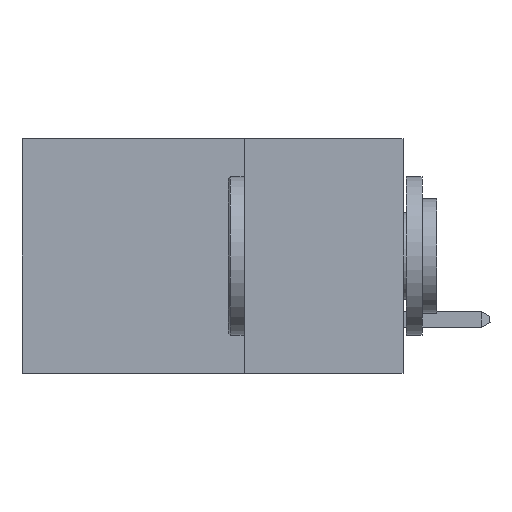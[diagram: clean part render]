
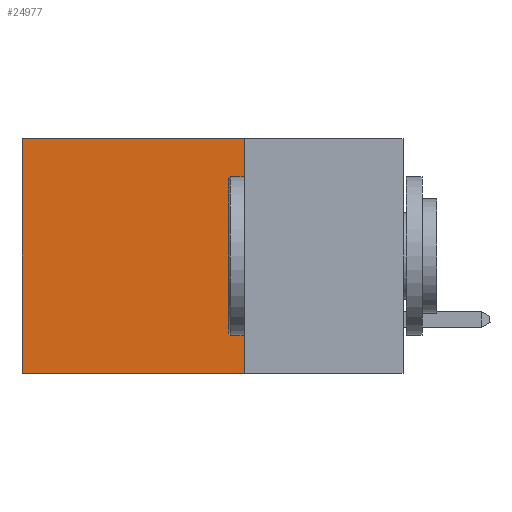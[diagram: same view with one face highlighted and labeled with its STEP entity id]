
A CAD part, left-side view. The second image highlights one B-rep face of the part: STEP entity #24977.
In plain terms, the highlighted planar face has unit normal (-1, 0, 0).
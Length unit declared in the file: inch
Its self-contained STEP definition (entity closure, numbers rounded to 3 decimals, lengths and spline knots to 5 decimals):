
#1694 = CARTESIAN_POINT ( 'NONE',  ( 0.2875, 0.6, 0. ) ) ;
#1926 = EDGE_CURVE ( 'NONE', #26159, #25544, #29488, .T. ) ;
#2100 = AXIS2_PLACEMENT_3D ( 'NONE', #13046, #10799, #15730 ) ;
#2441 = FACE_OUTER_BOUND ( 'NONE', #2463, .T. ) ;
#2463 = EDGE_LOOP ( 'NONE', ( #6213, #17209, #7531, #12561 ) ) ;
#2525 = PLANE ( 'NONE',  #2100 ) ;
#2778 = CARTESIAN_POINT ( 'NONE',  ( 0.2875, 0.6, -0.37 ) ) ;
#3217 = EDGE_CURVE ( 'NONE', #23354, #26159, #5115, .T. ) ;
#4455 = VECTOR ( 'NONE', #12534, 39.37008 ) ;
#4984 = EDGE_CURVE ( 'NONE', #25813, #25544, #27620, .T. ) ;
#5115 = LINE ( 'NONE', #22896, #5523 ) ;
#5523 = VECTOR ( 'NONE', #28778, 39.37008 ) ;
#6213 = ORIENTED_EDGE ( 'NONE', *, *, #4984, .T. ) ;
#7208 = EDGE_CURVE ( 'NONE', #23354, #25813, #27907, .T. ) ;
#7509 = VECTOR ( 'NONE', #21911, 39.37008 ) ;
#7531 = ORIENTED_EDGE ( 'NONE', *, *, #3217, .F. ) ;
#9911 = CARTESIAN_POINT ( 'NONE',  ( 0.2875, 0.6, 0. ) ) ;
#10799 = DIRECTION ( 'NONE',  ( 1., 0., 0. ) ) ;
#11289 = CARTESIAN_POINT ( 'NONE',  ( 0.2875, 0.25, -0.37 ) ) ;
#12534 = DIRECTION ( 'NONE',  ( 0., 1., 0. ) ) ;
#12561 = ORIENTED_EDGE ( 'NONE', *, *, #7208, .T. ) ;
#13046 = CARTESIAN_POINT ( 'NONE',  ( 0.2875, 0.25, 0. ) ) ;
#15730 = DIRECTION ( 'NONE',  ( 0., 0., -1. ) ) ;
#17209 = ORIENTED_EDGE ( 'NONE', *, *, #1926, .F. ) ;
#17318 = CARTESIAN_POINT ( 'NONE',  ( 0.2875, 0.25, 0. ) ) ;
#21911 = DIRECTION ( 'NONE',  ( 0., 0., -1. ) ) ;
#22896 = CARTESIAN_POINT ( 'NONE',  ( 0.2875, 0.25, 0. ) ) ;
#23354 = VERTEX_POINT ( 'NONE', #32966 ) ;
#24977 = ADVANCED_FACE ( 'NONE', ( #2441 ), #2525, .F. ) ;
#25544 = VERTEX_POINT ( 'NONE', #2778 ) ;
#25813 = VERTEX_POINT ( 'NONE', #1694 ) ;
#26159 = VERTEX_POINT ( 'NONE', #26625 ) ;
#26625 = CARTESIAN_POINT ( 'NONE',  ( 0.2875, 0.25, -0.37 ) ) ;
#27620 = LINE ( 'NONE', #9911, #7509 ) ;
#27907 = LINE ( 'NONE', #17318, #4455 ) ;
#28778 = DIRECTION ( 'NONE',  ( 0., 0., -1. ) ) ;
#29488 = LINE ( 'NONE', #11289, #34143 ) ;
#30047 = DIRECTION ( 'NONE',  ( 0., 1., 0. ) ) ;
#32966 = CARTESIAN_POINT ( 'NONE',  ( 0.2875, 0.25, 0. ) ) ;
#34143 = VECTOR ( 'NONE', #30047, 39.37008 ) ;
